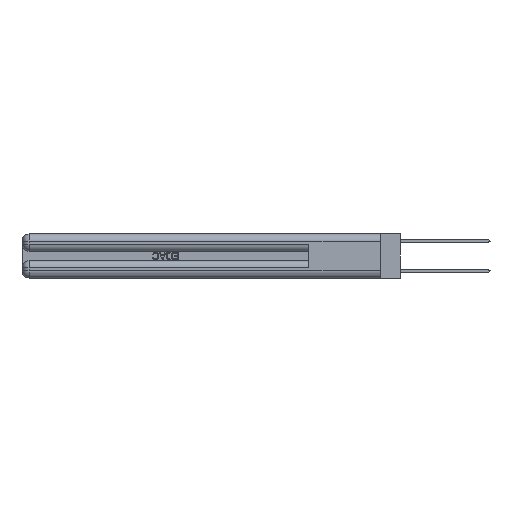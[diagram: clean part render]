
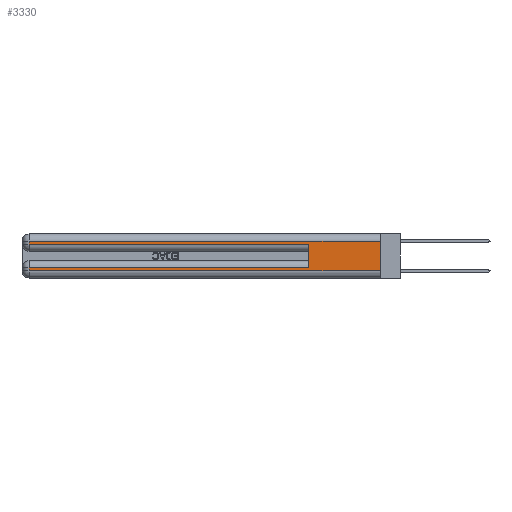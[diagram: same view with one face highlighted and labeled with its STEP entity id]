
A CAD part, left-side view. The second image highlights one B-rep face of the part: STEP entity #3330.
In plain terms, the highlighted planar face has unit normal (-1, 0, 0).
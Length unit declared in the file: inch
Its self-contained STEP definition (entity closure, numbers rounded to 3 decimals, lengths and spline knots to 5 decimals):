
#73 = LINE ( 'NONE', #7510, #7638 ) ;
#221 = CARTESIAN_POINT ( 'NONE',  ( 0., 0., 0.06 ) ) ;
#289 = CARTESIAN_POINT ( 'NONE',  ( 0., 0.6, 0.145 ) ) ;
#306 = EDGE_CURVE ( 'NONE', #25552, #850, #7927, .T. ) ;
#819 = ORIENTED_EDGE ( 'NONE', *, *, #8293, .T. ) ;
#850 = VERTEX_POINT ( 'NONE', #30004 ) ;
#1772 = LINE ( 'NONE', #4085, #21467 ) ;
#2097 = CARTESIAN_POINT ( 'NONE',  ( 0., 2.94, 0.06 ) ) ;
#2336 = CARTESIAN_POINT ( 'NONE',  ( 0., 0., 0.31 ) ) ;
#3232 = VERTEX_POINT ( 'NONE', #9164 ) ;
#3330 = ADVANCED_FACE ( 'NONE', ( #25121 ), #27582, .F. ) ;
#3906 = DIRECTION ( 'NONE',  ( 0., 0., -1. ) ) ;
#4085 = CARTESIAN_POINT ( 'NONE',  ( 0., 0., 0.37 ) ) ;
#4244 = CARTESIAN_POINT ( 'NONE',  ( 0., 0., 0.085 ) ) ;
#4966 = VECTOR ( 'NONE', #17842, 39.37008 ) ;
#5031 = DIRECTION ( 'NONE',  ( 0., 0., -1. ) ) ;
#5685 = EDGE_LOOP ( 'NONE', ( #29212, #819, #24095, #6936, #29594, #25126, #26138, #13420 ) ) ;
#5817 = CARTESIAN_POINT ( 'NONE',  ( 0., 2.94, 0.285 ) ) ;
#6936 = ORIENTED_EDGE ( 'NONE', *, *, #306, .T. ) ;
#7328 = VECTOR ( 'NONE', #3906, 39.37008 ) ;
#7510 = CARTESIAN_POINT ( 'NONE',  ( 0., 2.94, 0.37 ) ) ;
#7638 = VECTOR ( 'NONE', #5031, 39.37008 ) ;
#7927 = LINE ( 'NONE', #27445, #4966 ) ;
#8049 = VECTOR ( 'NONE', #19865, 39.37008 ) ;
#8293 = EDGE_CURVE ( 'NONE', #13844, #14614, #19565, .T. ) ;
#8374 = VERTEX_POINT ( 'NONE', #16865 ) ;
#8740 = DIRECTION ( 'NONE',  ( 0., 0., -1. ) ) ;
#9164 = CARTESIAN_POINT ( 'NONE',  ( 0., 0.6, 0.085 ) ) ;
#10114 = EDGE_CURVE ( 'NONE', #8374, #17615, #73, .T. ) ;
#10442 = EDGE_CURVE ( 'NONE', #13844, #24053, #1772, .T. ) ;
#10452 = EDGE_CURVE ( 'NONE', #3232, #8374, #15716, .T. ) ;
#10630 = CARTESIAN_POINT ( 'NONE',  ( 0., 2.94, 0.31 ) ) ;
#10873 = EDGE_CURVE ( 'NONE', #14614, #25552, #30073, .T. ) ;
#11772 = LINE ( 'NONE', #289, #23689 ) ;
#12593 = AXIS2_PLACEMENT_3D ( 'NONE', #25262, #15492, #17682 ) ;
#12988 = EDGE_CURVE ( 'NONE', #17615, #24053, #18992, .T. ) ;
#13420 = ORIENTED_EDGE ( 'NONE', *, *, #12988, .T. ) ;
#13844 = VERTEX_POINT ( 'NONE', #2336 ) ;
#13867 = EDGE_CURVE ( 'NONE', #3232, #850, #11772, .T. ) ;
#14614 = VERTEX_POINT ( 'NONE', #10630 ) ;
#15492 = DIRECTION ( 'NONE',  ( 1., 0., 0. ) ) ;
#15716 = LINE ( 'NONE', #4244, #25428 ) ;
#16865 = CARTESIAN_POINT ( 'NONE',  ( 0., 2.94, 0.085 ) ) ;
#17537 = CARTESIAN_POINT ( 'NONE',  ( 0., 0., 0.31 ) ) ;
#17615 = VERTEX_POINT ( 'NONE', #2097 ) ;
#17682 = DIRECTION ( 'NONE',  ( 0., 0., -1. ) ) ;
#17842 = DIRECTION ( 'NONE',  ( 0., -1., 0. ) ) ;
#18915 = DIRECTION ( 'NONE',  ( 0., 0., 1. ) ) ;
#18992 = LINE ( 'NONE', #221, #27876 ) ;
#19565 = LINE ( 'NONE', #17537, #8049 ) ;
#19865 = DIRECTION ( 'NONE',  ( 0., 1., 0. ) ) ;
#21467 = VECTOR ( 'NONE', #8740, 39.37008 ) ;
#22661 = CARTESIAN_POINT ( 'NONE',  ( 0., 2.94, 0.37 ) ) ;
#22993 = DIRECTION ( 'NONE',  ( 0., 1., 0. ) ) ;
#23689 = VECTOR ( 'NONE', #18915, 39.37008 ) ;
#24053 = VERTEX_POINT ( 'NONE', #24254 ) ;
#24095 = ORIENTED_EDGE ( 'NONE', *, *, #10873, .T. ) ;
#24254 = CARTESIAN_POINT ( 'NONE',  ( 0., 0., 0.06 ) ) ;
#25121 = FACE_OUTER_BOUND ( 'NONE', #5685, .T. ) ;
#25126 = ORIENTED_EDGE ( 'NONE', *, *, #10452, .T. ) ;
#25262 = CARTESIAN_POINT ( 'NONE',  ( 0., 0., 0.37 ) ) ;
#25428 = VECTOR ( 'NONE', #22993, 39.37008 ) ;
#25552 = VERTEX_POINT ( 'NONE', #5817 ) ;
#26138 = ORIENTED_EDGE ( 'NONE', *, *, #10114, .T. ) ;
#27445 = CARTESIAN_POINT ( 'NONE',  ( 0., 0., 0.285 ) ) ;
#27582 = PLANE ( 'NONE',  #12593 ) ;
#27876 = VECTOR ( 'NONE', #28423, 39.37008 ) ;
#28423 = DIRECTION ( 'NONE',  ( 0., -1., 0. ) ) ;
#29212 = ORIENTED_EDGE ( 'NONE', *, *, #10442, .F. ) ;
#29594 = ORIENTED_EDGE ( 'NONE', *, *, #13867, .F. ) ;
#30004 = CARTESIAN_POINT ( 'NONE',  ( 0., 0.6, 0.285 ) ) ;
#30073 = LINE ( 'NONE', #22661, #7328 ) ;
